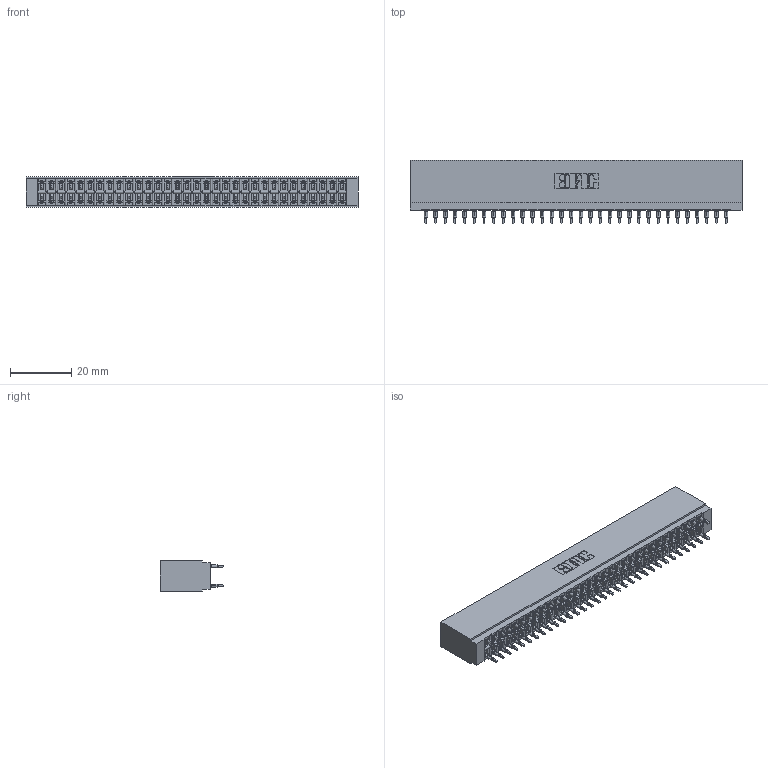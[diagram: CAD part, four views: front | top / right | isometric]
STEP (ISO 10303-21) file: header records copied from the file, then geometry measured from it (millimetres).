
FILE_DESCRIPTION (( 'STEP AP203' ), '1' );
FILE_NAME ('746-064-560-201.STEP', '2026-03-04T13:59:34', ( '' ), ( '' ), 'SwSTEP 2.0', 'SolidWorks 2023', '' );
FILE_SCHEMA (( 'CONFIG_CONTROL_DESIGN' ));
Length unit declared in the file: millimetre
Products named in the file (3): 746-292-001_560; 746-064-560-201; 746 Part_.515 Slot Depth - 01
Assembly tree (65 placements, depth 2):
  746-064-560-201
    746 Part_.515 Slot Depth - 01
    746-292-001_560  x64
Bounding box: 108.84 x 20.82 x 9.91 mm (x, y, z)
Volume: 11952.5 mm3; surface area: 20035.8 mm2
Topology: 65 solids, 65 shells, 6145 faces, 17095 edges, 10959 vertices
Faces by surface type: plane 3063, cylinder 1418, bspline 1280, torus 384
Entity records: 50980 total; most frequent: CARTESIAN_POINT 10219, ORIENTED_EDGE 8738, DIRECTION 7319, EDGE_CURVE 4369, LINE 3857, VECTOR 3857, VERTEX_POINT 2895, AXIS2_PLACEMENT_3D 1731
